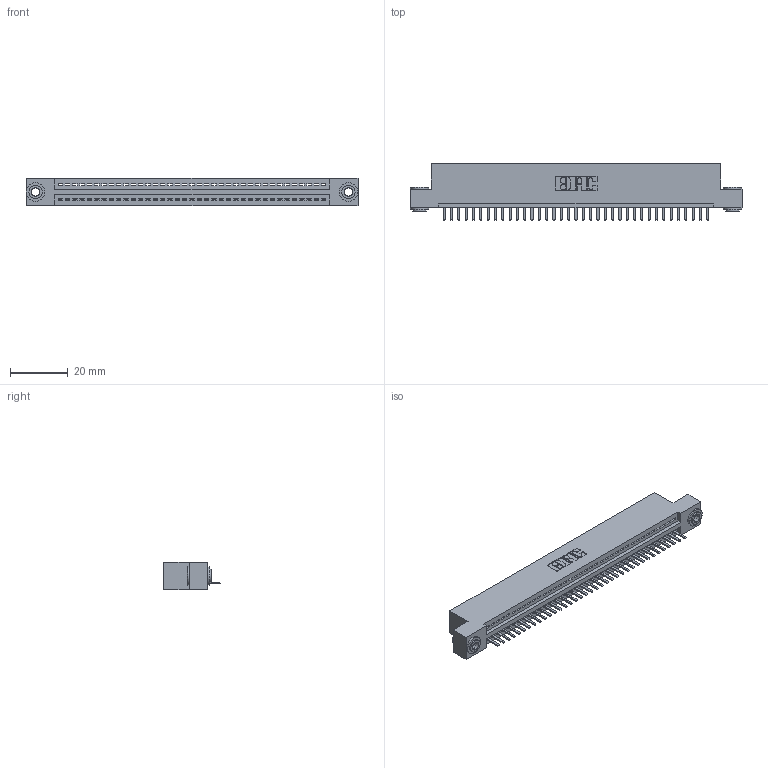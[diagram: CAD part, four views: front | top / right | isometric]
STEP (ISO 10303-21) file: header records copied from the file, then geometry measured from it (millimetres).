
FILE_DESCRIPTION (( 'STEP AP203' ), '1' );
FILE_NAME ('345-037-520-103.STEP', '2019-10-08T00:24:41', ( '' ), ( '' ), 'SwSTEP 2.0', 'SolidWorks 2016', '' );
FILE_SCHEMA (( 'CONFIG_CONTROL_DESIGN' ));
Length unit declared in the file: inch
Products named in the file (4): 345 Part_Flush Mounting Lugs - 0.156 Dia-TH; 345-292-001_345-293-120; 345-037-520-103; 345-250-002_345-250-002-102
Assembly tree (40 placements, depth 2):
  345-037-520-103
    345 Part_Flush Mounting Lugs - 0.156 Dia-TH
    345-292-001_345-293-120  x37
    345-250-002_345-250-002-102  x2
Bounding box: 115.19 x 19.68 x 9.4 mm (x, y, z)
Volume: 10812.8 mm3; surface area: 14167.5 mm2
Topology: 40 solids, 40 shells, 2458 faces, 7225 edges, 4714 vertices
Faces by surface type: plane 1644, cylinder 806, cone 8
Entity records: 29284 total; most frequent: CARTESIAN_POINT 5062, ORIENTED_EDGE 5014, DIRECTION 4447, EDGE_CURVE 2507, LINE 2199, VECTOR 2199, VERTEX_POINT 1666, AXIS2_PLACEMENT_3D 1124
